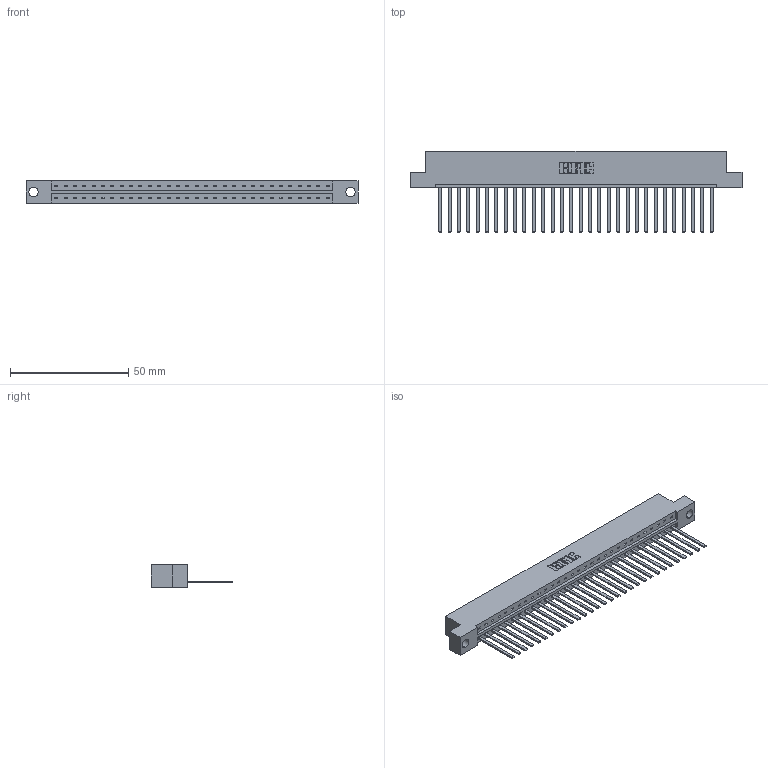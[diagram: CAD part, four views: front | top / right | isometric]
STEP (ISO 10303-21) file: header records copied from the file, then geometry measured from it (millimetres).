
FILE_DESCRIPTION (( 'STEP AP203' ), '1' );
FILE_NAME ('833-030-544-104.STEP', '2020-06-02T13:41:27', ( '' ), ( '' ), 'SwSTEP 2.0', 'SolidWorks 2020', '' );
FILE_SCHEMA (( 'CONFIG_CONTROL_DESIGN' ));
Length unit declared in the file: inch
Products named in the file (3): 345-292-001_345-293-144; 833-030-544-104; 833 Part_Flush - .156 Dia - TH
Assembly tree (31 placements, depth 2):
  833-030-544-104
    833 Part_Flush - .156 Dia - TH
    345-292-001_345-293-144  x30
Bounding box: 140.41 x 34.3 x 9.4 mm (x, y, z)
Volume: 14285.7 mm3; surface area: 16303.5 mm2
Topology: 31 solids, 31 shells, 1674 faces, 5051 edges, 3326 vertices
Faces by surface type: plane 1210, cylinder 464
Entity records: 19711 total; most frequent: CARTESIAN_POINT 3408, ORIENTED_EDGE 3374, DIRECTION 2895, EDGE_CURVE 1687, LINE 1563, VECTOR 1563, VERTEX_POINT 1122, AXIS2_PLACEMENT_3D 666
